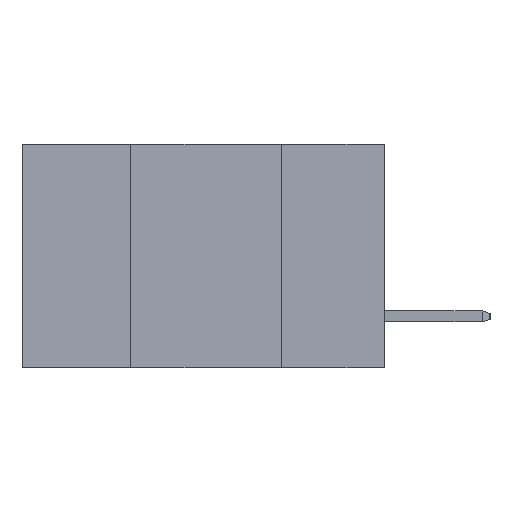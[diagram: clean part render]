
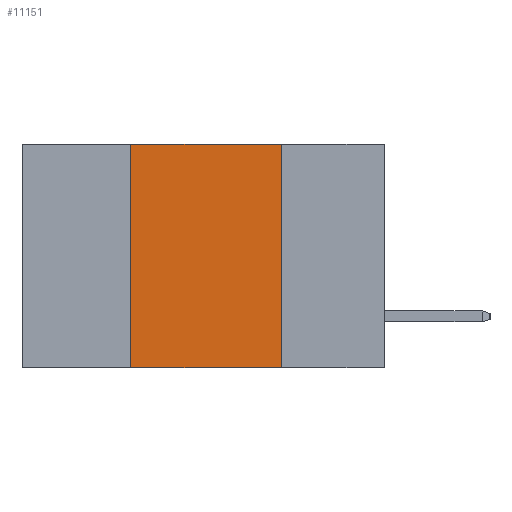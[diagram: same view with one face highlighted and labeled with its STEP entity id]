
A CAD part, left-side view. The second image highlights one B-rep face of the part: STEP entity #11151.
In plain terms, the highlighted planar face has unit normal (-1, 0, 0).
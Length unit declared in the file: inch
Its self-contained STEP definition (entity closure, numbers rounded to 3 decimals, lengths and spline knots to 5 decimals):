
#151 = VERTEX_POINT ( 'NONE', #17823 ) ;
#279 = PLANE ( 'NONE',  #16669 ) ;
#399 = EDGE_CURVE ( 'NONE', #22590, #28040, #20264, .T. ) ;
#1965 = DIRECTION ( 'NONE',  ( 0., -1., 0. ) ) ;
#2435 = LINE ( 'NONE', #29224, #8081 ) ;
#2690 = CARTESIAN_POINT ( 'NONE',  ( 0., 0.6, 0. ) ) ;
#3163 = FACE_OUTER_BOUND ( 'NONE', #22690, .T. ) ;
#3744 = CARTESIAN_POINT ( 'NONE',  ( 0., 0.6, 0. ) ) ;
#4452 = CARTESIAN_POINT ( 'NONE',  ( 0., 0.42, 0. ) ) ;
#5103 = DIRECTION ( 'NONE',  ( 1., 0., 0. ) ) ;
#5990 = EDGE_CURVE ( 'NONE', #29742, #151, #28987, .T. ) ;
#6081 = VECTOR ( 'NONE', #12299, 39.37008 ) ;
#7766 = CARTESIAN_POINT ( 'NONE',  ( 0., 0.17, 0. ) ) ;
#8081 = VECTOR ( 'NONE', #13206, 39.37008 ) ;
#10663 = VECTOR ( 'NONE', #25116, 39.37008 ) ;
#10795 = EDGE_CURVE ( 'NONE', #29742, #22590, #2435, .T. ) ;
#11151 = ADVANCED_FACE ( 'NONE', ( #3163 ), #279, .F. ) ;
#12299 = DIRECTION ( 'NONE',  ( 0., 0., -1. ) ) ;
#12348 = EDGE_CURVE ( 'NONE', #28040, #151, #23883, .T. ) ;
#13206 = DIRECTION ( 'NONE',  ( 0., 0., 1. ) ) ;
#14145 = CARTESIAN_POINT ( 'NONE',  ( 0., 0.42, -0.37 ) ) ;
#14187 = VECTOR ( 'NONE', #1965, 39.37008 ) ;
#15752 = ORIENTED_EDGE ( 'NONE', *, *, #12348, .F. ) ;
#16669 = AXIS2_PLACEMENT_3D ( 'NONE', #2690, #5103, #21428 ) ;
#17189 = ORIENTED_EDGE ( 'NONE', *, *, #399, .F. ) ;
#17823 = CARTESIAN_POINT ( 'NONE',  ( 0., 0.17, -0.37 ) ) ;
#20264 = LINE ( 'NONE', #3744, #14187 ) ;
#21428 = DIRECTION ( 'NONE',  ( 0., 0., -1. ) ) ;
#21467 = CARTESIAN_POINT ( 'NONE',  ( 0., 0.17, 0. ) ) ;
#22590 = VERTEX_POINT ( 'NONE', #4452 ) ;
#22690 = EDGE_LOOP ( 'NONE', ( #15752, #17189, #29309, #25173 ) ) ;
#23883 = LINE ( 'NONE', #21467, #6081 ) ;
#25116 = DIRECTION ( 'NONE',  ( 0., -1., 0. ) ) ;
#25173 = ORIENTED_EDGE ( 'NONE', *, *, #5990, .T. ) ;
#25183 = CARTESIAN_POINT ( 'NONE',  ( 0., 0.6, -0.37 ) ) ;
#28040 = VERTEX_POINT ( 'NONE', #7766 ) ;
#28987 = LINE ( 'NONE', #25183, #10663 ) ;
#29224 = CARTESIAN_POINT ( 'NONE',  ( 0., 0.42, 0. ) ) ;
#29309 = ORIENTED_EDGE ( 'NONE', *, *, #10795, .F. ) ;
#29742 = VERTEX_POINT ( 'NONE', #14145 ) ;
